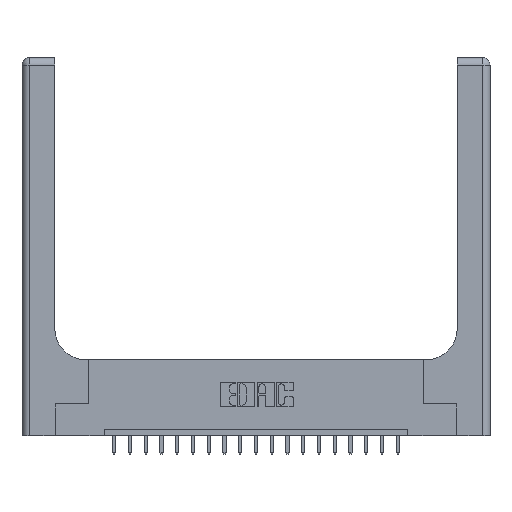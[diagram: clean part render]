
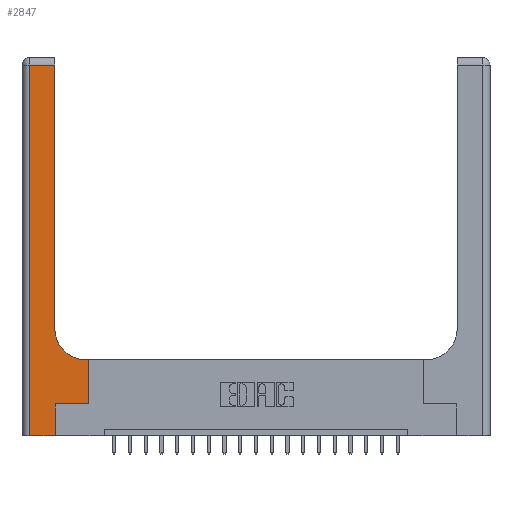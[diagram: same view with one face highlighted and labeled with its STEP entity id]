
A CAD part, top view. The second image highlights one B-rep face of the part: STEP entity #2847.
In plain terms, the highlighted planar face has unit normal (0, 0, 1).
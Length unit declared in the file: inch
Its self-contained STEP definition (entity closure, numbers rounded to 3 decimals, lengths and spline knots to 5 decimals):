
#667 = CARTESIAN_POINT ( 'NONE',  ( 0.265, 0.25, 0.37 ) ) ;
#976 = DIRECTION ( 'NONE',  ( -1., 0., 0. ) ) ;
#1282 = CARTESIAN_POINT ( 'NONE',  ( 0.06, 2.94, 0.37 ) ) ;
#1350 = VERTEX_POINT ( 'NONE', #14205 ) ;
#1351 = CARTESIAN_POINT ( 'NONE',  ( 0.26, 2.94, 0.37 ) ) ;
#1502 = CIRCLE ( 'NONE', #13437, 0.25 ) ;
#1505 = VECTOR ( 'NONE', #5533, 39.37008 ) ;
#1539 = LINE ( 'NONE', #9332, #11666 ) ;
#1727 = VERTEX_POINT ( 'NONE', #18410 ) ;
#2460 = VECTOR ( 'NONE', #11925, 39.37008 ) ;
#2478 = VECTOR ( 'NONE', #7228, 39.37008 ) ;
#2847 = ADVANCED_FACE ( 'NONE', ( #11590 ), #5067, .F. ) ;
#2921 = ORIENTED_EDGE ( 'NONE', *, *, #19322, .T. ) ;
#3317 = EDGE_CURVE ( 'NONE', #1350, #1727, #10407, .T. ) ;
#4340 = ORIENTED_EDGE ( 'NONE', *, *, #11323, .T. ) ;
#4670 = CARTESIAN_POINT ( 'NONE',  ( 0.06, 0., 0.37 ) ) ;
#5067 = PLANE ( 'NONE',  #13540 ) ;
#5533 = DIRECTION ( 'NONE',  ( 0., 1., 0. ) ) ;
#5595 = CARTESIAN_POINT ( 'NONE',  ( 0.06, 3., 0.37 ) ) ;
#5862 = EDGE_CURVE ( 'NONE', #11335, #8133, #17008, .T. ) ;
#5867 = CARTESIAN_POINT ( 'NONE',  ( 0.265, 0.25, 0.37 ) ) ;
#5933 = VERTEX_POINT ( 'NONE', #4670 ) ;
#5947 = CARTESIAN_POINT ( 'NONE',  ( 0.26, 3., 0.37 ) ) ;
#7228 = DIRECTION ( 'NONE',  ( 1., 0., 0. ) ) ;
#7268 = LINE ( 'NONE', #5595, #2460 ) ;
#7536 = ORIENTED_EDGE ( 'NONE', *, *, #3317, .T. ) ;
#7660 = VECTOR ( 'NONE', #17421, 39.37008 ) ;
#7676 = CARTESIAN_POINT ( 'NONE',  ( 0.265, 0., 0.37 ) ) ;
#7894 = CARTESIAN_POINT ( 'NONE',  ( 0.265, 0., 0.37 ) ) ;
#8133 = VERTEX_POINT ( 'NONE', #5867 ) ;
#8531 = EDGE_CURVE ( 'NONE', #1727, #10601, #1502, .T. ) ;
#8566 = ORIENTED_EDGE ( 'NONE', *, *, #13069, .T. ) ;
#9060 = DIRECTION ( 'NONE',  ( 0., 0., -1. ) ) ;
#9332 = CARTESIAN_POINT ( 'NONE',  ( 0., 2.94, 0.37 ) ) ;
#9727 = CARTESIAN_POINT ( 'NONE',  ( 0., 3., 0.37 ) ) ;
#9906 = ORIENTED_EDGE ( 'NONE', *, *, #10885, .T. ) ;
#10407 = LINE ( 'NONE', #19653, #12589 ) ;
#10601 = VERTEX_POINT ( 'NONE', #20426 ) ;
#10714 = LINE ( 'NONE', #5947, #1505 ) ;
#10885 = EDGE_CURVE ( 'NONE', #8133, #16069, #16348, .T. ) ;
#10898 = LINE ( 'NONE', #14328, #19893 ) ;
#11323 = EDGE_CURVE ( 'NONE', #5933, #11335, #10898, .T. ) ;
#11335 = VERTEX_POINT ( 'NONE', #7894 ) ;
#11590 = FACE_OUTER_BOUND ( 'NONE', #18487, .T. ) ;
#11637 = ORIENTED_EDGE ( 'NONE', *, *, #5862, .T. ) ;
#11666 = VECTOR ( 'NONE', #18861, 39.37008 ) ;
#11925 = DIRECTION ( 'NONE',  ( 0., -1., 0. ) ) ;
#12457 = DIRECTION ( 'NONE',  ( 0., 1., 0. ) ) ;
#12565 = DIRECTION ( 'NONE',  ( 1., 0., 0. ) ) ;
#12589 = VECTOR ( 'NONE', #976, 39.37008 ) ;
#13052 = DIRECTION ( 'NONE',  ( -1., 0., 0. ) ) ;
#13069 = EDGE_CURVE ( 'NONE', #16069, #1350, #14130, .T. ) ;
#13437 = AXIS2_PLACEMENT_3D ( 'NONE', #15192, #9060, #19953 ) ;
#13445 = VERTEX_POINT ( 'NONE', #1282 ) ;
#13540 = AXIS2_PLACEMENT_3D ( 'NONE', #9727, #17896, #13052 ) ;
#14130 = LINE ( 'NONE', #20465, #7660 ) ;
#14205 = CARTESIAN_POINT ( 'NONE',  ( 0.528, 0.6, 0.37 ) ) ;
#14328 = CARTESIAN_POINT ( 'NONE',  ( 0., 0., 0.37 ) ) ;
#14403 = EDGE_CURVE ( 'NONE', #16256, #13445, #1539, .T. ) ;
#15192 = CARTESIAN_POINT ( 'NONE',  ( 0.51, 0.85, 0.37 ) ) ;
#16069 = VERTEX_POINT ( 'NONE', #16917 ) ;
#16256 = VERTEX_POINT ( 'NONE', #1351 ) ;
#16348 = LINE ( 'NONE', #667, #2478 ) ;
#16656 = ORIENTED_EDGE ( 'NONE', *, *, #8531, .T. ) ;
#16917 = CARTESIAN_POINT ( 'NONE',  ( 0.528, 0.25, 0.37 ) ) ;
#17008 = LINE ( 'NONE', #7676, #17744 ) ;
#17421 = DIRECTION ( 'NONE',  ( 0., 1., 0. ) ) ;
#17422 = ORIENTED_EDGE ( 'NONE', *, *, #14403, .T. ) ;
#17744 = VECTOR ( 'NONE', #12457, 39.37008 ) ;
#17896 = DIRECTION ( 'NONE',  ( 0., 0., -1. ) ) ;
#18008 = ORIENTED_EDGE ( 'NONE', *, *, #19950, .T. ) ;
#18410 = CARTESIAN_POINT ( 'NONE',  ( 0.51, 0.6, 0.37 ) ) ;
#18487 = EDGE_LOOP ( 'NONE', ( #18008, #17422, #2921, #4340, #11637, #9906, #8566, #7536, #16656 ) ) ;
#18861 = DIRECTION ( 'NONE',  ( -1., 0., 0. ) ) ;
#19322 = EDGE_CURVE ( 'NONE', #13445, #5933, #7268, .T. ) ;
#19653 = CARTESIAN_POINT ( 'NONE',  ( 0.26, 0.6, 0.37 ) ) ;
#19893 = VECTOR ( 'NONE', #12565, 39.37008 ) ;
#19950 = EDGE_CURVE ( 'NONE', #10601, #16256, #10714, .T. ) ;
#19953 = DIRECTION ( 'NONE',  ( 1., 0., 0. ) ) ;
#20426 = CARTESIAN_POINT ( 'NONE',  ( 0.26, 0.85, 0.37 ) ) ;
#20465 = CARTESIAN_POINT ( 'NONE',  ( 0.528, 0.25, 0.37 ) ) ;
